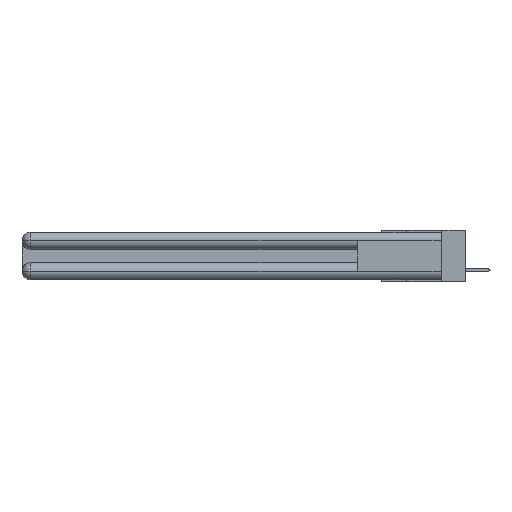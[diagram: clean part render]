
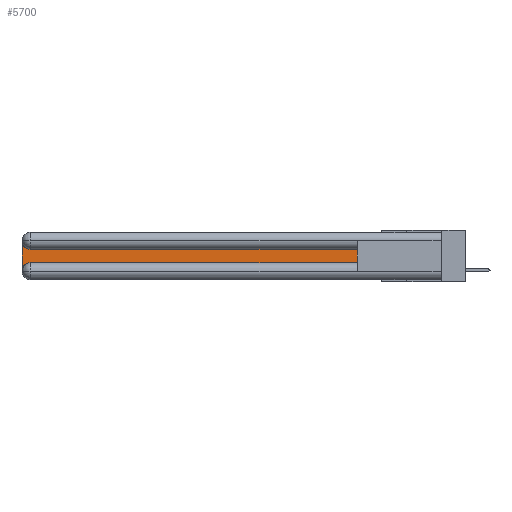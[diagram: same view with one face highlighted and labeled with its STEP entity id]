
A CAD part, left-side view. The second image highlights one B-rep face of the part: STEP entity #5700.
In plain terms, the highlighted planar face has unit normal (-1, 0, 0).
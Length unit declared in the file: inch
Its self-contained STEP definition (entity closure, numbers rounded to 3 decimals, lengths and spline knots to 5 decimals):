
#429 = DIRECTION ( 'NONE',  ( 1., 0., 0. ) ) ;
#478 = CARTESIAN_POINT ( 'NONE',  ( 0.075, 3., -0.2775 ) ) ;
#1356 = LINE ( 'NONE', #2773, #16155 ) ;
#1689 = CARTESIAN_POINT ( 'NONE',  ( 0.075, 0.6, -0.1225 ) ) ;
#2325 = EDGE_CURVE ( 'NONE', #6551, #28954, #21738, .T. ) ;
#2468 = VERTEX_POINT ( 'NONE', #478 ) ;
#2773 = CARTESIAN_POINT ( 'NONE',  ( 0.075, 0.6, -0.1225 ) ) ;
#3507 = CARTESIAN_POINT ( 'NONE',  ( 0.075, 3., -0.1225 ) ) ;
#5700 = ADVANCED_FACE ( 'NONE', ( #18442 ), #6012, .F. ) ;
#6012 = PLANE ( 'NONE',  #8911 ) ;
#6313 = AXIS2_PLACEMENT_3D ( 'NONE', #15057, #429, #17878 ) ;
#6551 = VERTEX_POINT ( 'NONE', #17108 ) ;
#7133 = DIRECTION ( 'NONE',  ( 0., 0., 1. ) ) ;
#7820 = ORIENTED_EDGE ( 'NONE', *, *, #2325, .T. ) ;
#8911 = AXIS2_PLACEMENT_3D ( 'NONE', #3507, #28303, #13437 ) ;
#9410 = VECTOR ( 'NONE', #28341, 39.37008 ) ;
#12677 = CARTESIAN_POINT ( 'NONE',  ( 0.075, 2.94, -0.1225 ) ) ;
#12693 = DIRECTION ( 'NONE',  ( 0., 1., 0. ) ) ;
#13045 = EDGE_CURVE ( 'NONE', #2468, #22870, #28510, .T. ) ;
#13437 = DIRECTION ( 'NONE',  ( 0., 0., -1. ) ) ;
#14423 = DIRECTION ( 'NONE',  ( 0., -1., 0. ) ) ;
#14525 = DIRECTION ( 'NONE',  ( 1., 0., 0. ) ) ;
#14539 = ORIENTED_EDGE ( 'NONE', *, *, #24058, .T. ) ;
#15057 = CARTESIAN_POINT ( 'NONE',  ( 0.075, 2.94, -0.2775 ) ) ;
#15143 = ORIENTED_EDGE ( 'NONE', *, *, #18368, .T. ) ;
#15892 = CARTESIAN_POINT ( 'NONE',  ( 0.075, 3., -0.2175 ) ) ;
#16155 = VECTOR ( 'NONE', #12693, 39.37008 ) ;
#16382 = EDGE_CURVE ( 'NONE', #18805, #17445, #28634, .T. ) ;
#16416 = AXIS2_PLACEMENT_3D ( 'NONE', #32202, #14525, #29584 ) ;
#16421 = CARTESIAN_POINT ( 'NONE',  ( 0.075, 3., -0.0625 ) ) ;
#17108 = CARTESIAN_POINT ( 'NONE',  ( 0.075, 0.6, -0.2175 ) ) ;
#17445 = VERTEX_POINT ( 'NONE', #16421 ) ;
#17878 = DIRECTION ( 'NONE',  ( 0., 0., -1. ) ) ;
#17909 = ORIENTED_EDGE ( 'NONE', *, *, #13045, .T. ) ;
#18368 = EDGE_CURVE ( 'NONE', #17445, #2468, #18757, .T. ) ;
#18442 = FACE_OUTER_BOUND ( 'NONE', #32157, .T. ) ;
#18757 = LINE ( 'NONE', #15892, #9410 ) ;
#18805 = VERTEX_POINT ( 'NONE', #12677 ) ;
#18846 = VECTOR ( 'NONE', #14423, 39.37008 ) ;
#19444 = ORIENTED_EDGE ( 'NONE', *, *, #16382, .T. ) ;
#19656 = CARTESIAN_POINT ( 'NONE',  ( 0.075, 0.6, -0.2175 ) ) ;
#21738 = LINE ( 'NONE', #19656, #24449 ) ;
#22870 = VERTEX_POINT ( 'NONE', #24330 ) ;
#23454 = ORIENTED_EDGE ( 'NONE', *, *, #29231, .T. ) ;
#24058 = EDGE_CURVE ( 'NONE', #28954, #18805, #1356, .T. ) ;
#24330 = CARTESIAN_POINT ( 'NONE',  ( 0.075, 2.94, -0.2175 ) ) ;
#24449 = VECTOR ( 'NONE', #7133, 39.37008 ) ;
#24634 = LINE ( 'NONE', #27097, #18846 ) ;
#27097 = CARTESIAN_POINT ( 'NONE',  ( 0.075, 0.6, -0.2175 ) ) ;
#28303 = DIRECTION ( 'NONE',  ( 1., 0., 0. ) ) ;
#28341 = DIRECTION ( 'NONE',  ( 0., 0., -1. ) ) ;
#28510 = CIRCLE ( 'NONE', #6313, 0.06 ) ;
#28634 = CIRCLE ( 'NONE', #16416, 0.06 ) ;
#28954 = VERTEX_POINT ( 'NONE', #1689 ) ;
#29231 = EDGE_CURVE ( 'NONE', #22870, #6551, #24634, .T. ) ;
#29584 = DIRECTION ( 'NONE',  ( 0., 0., -1. ) ) ;
#32157 = EDGE_LOOP ( 'NONE', ( #14539, #19444, #15143, #17909, #23454, #7820 ) ) ;
#32202 = CARTESIAN_POINT ( 'NONE',  ( 0.075, 2.94, -0.0625 ) ) ;
